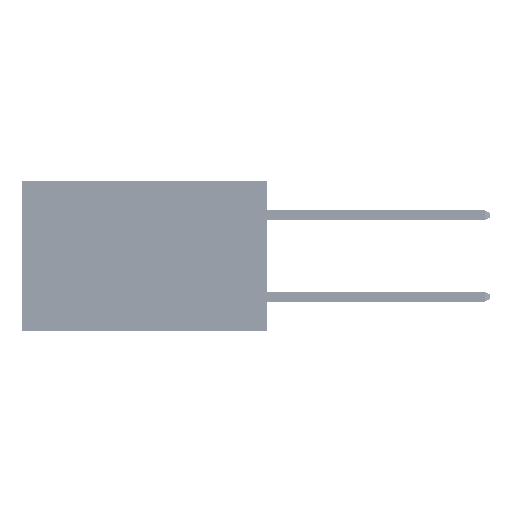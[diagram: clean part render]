
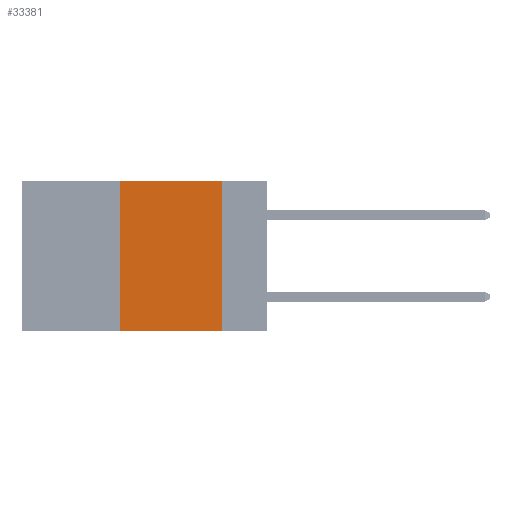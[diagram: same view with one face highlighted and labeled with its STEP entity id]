
A CAD part, left-side view. The second image highlights one B-rep face of the part: STEP entity #33381.
In plain terms, the highlighted planar face has unit normal (-1, 0, 0).
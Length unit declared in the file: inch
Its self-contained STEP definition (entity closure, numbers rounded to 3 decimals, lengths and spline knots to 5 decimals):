
#1924 = CARTESIAN_POINT ( 'NONE',  ( 0., 0.6, -0.37 ) ) ;
#2771 = CARTESIAN_POINT ( 'NONE',  ( 0., 0.11, -0.37 ) ) ;
#5874 = LINE ( 'NONE', #45943, #46791 ) ;
#6905 = DIRECTION ( 'NONE',  ( 0., 0., -1. ) ) ;
#9052 = VECTOR ( 'NONE', #23801, 39.37008 ) ;
#10720 = PLANE ( 'NONE',  #13841 ) ;
#12154 = CARTESIAN_POINT ( 'NONE',  ( 0., 0.6, 0. ) ) ;
#13841 = AXIS2_PLACEMENT_3D ( 'NONE', #38304, #42426, #18183 ) ;
#14223 = ORIENTED_EDGE ( 'NONE', *, *, #25910, .F. ) ;
#15826 = LINE ( 'NONE', #40252, #9052 ) ;
#15982 = CARTESIAN_POINT ( 'NONE',  ( 0., 0.11, 0. ) ) ;
#16818 = DIRECTION ( 'NONE',  ( 0., -1., 0. ) ) ;
#18183 = DIRECTION ( 'NONE',  ( 0., 0., -1. ) ) ;
#20371 = ORIENTED_EDGE ( 'NONE', *, *, #25071, .T. ) ;
#21500 = VERTEX_POINT ( 'NONE', #40457 ) ;
#22885 = ORIENTED_EDGE ( 'NONE', *, *, #46623, .F. ) ;
#22895 = VERTEX_POINT ( 'NONE', #15982 ) ;
#23801 = DIRECTION ( 'NONE',  ( 0., 0., 1. ) ) ;
#25071 = EDGE_CURVE ( 'NONE', #35839, #27699, #50020, .T. ) ;
#25885 = VECTOR ( 'NONE', #16818, 39.37008 ) ;
#25910 = EDGE_CURVE ( 'NONE', #35839, #21500, #15826, .T. ) ;
#26463 = VECTOR ( 'NONE', #41407, 39.37008 ) ;
#27699 = VERTEX_POINT ( 'NONE', #2771 ) ;
#30917 = EDGE_LOOP ( 'NONE', ( #45775, #22885, #14223, #20371 ) ) ;
#32701 = FACE_OUTER_BOUND ( 'NONE', #30917, .T. ) ;
#33381 = ADVANCED_FACE ( 'NONE', ( #32701 ), #10720, .F. ) ;
#34482 = EDGE_CURVE ( 'NONE', #22895, #27699, #5874, .T. ) ;
#35839 = VERTEX_POINT ( 'NONE', #50613 ) ;
#38304 = CARTESIAN_POINT ( 'NONE',  ( 0., 0.6, 0. ) ) ;
#40252 = CARTESIAN_POINT ( 'NONE',  ( 0., 0.36, 0. ) ) ;
#40457 = CARTESIAN_POINT ( 'NONE',  ( 0., 0.36, 0. ) ) ;
#41407 = DIRECTION ( 'NONE',  ( 0., -1., 0. ) ) ;
#42426 = DIRECTION ( 'NONE',  ( 1., 0., 0. ) ) ;
#45775 = ORIENTED_EDGE ( 'NONE', *, *, #34482, .F. ) ;
#45943 = CARTESIAN_POINT ( 'NONE',  ( 0., 0.11, 0. ) ) ;
#46623 = EDGE_CURVE ( 'NONE', #21500, #22895, #49421, .T. ) ;
#46791 = VECTOR ( 'NONE', #6905, 39.37008 ) ;
#49421 = LINE ( 'NONE', #12154, #25885 ) ;
#50020 = LINE ( 'NONE', #1924, #26463 ) ;
#50613 = CARTESIAN_POINT ( 'NONE',  ( 0., 0.36, -0.37 ) ) ;
